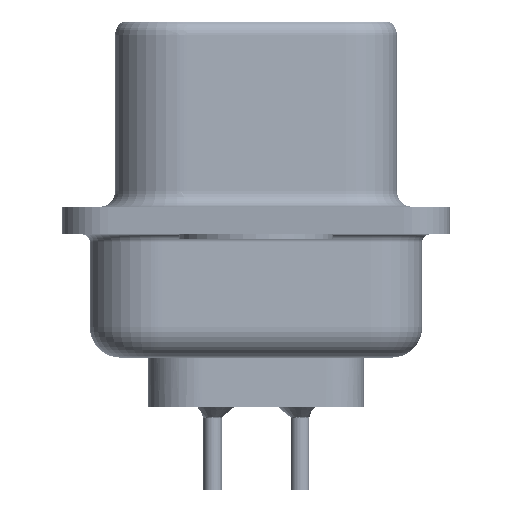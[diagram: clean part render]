
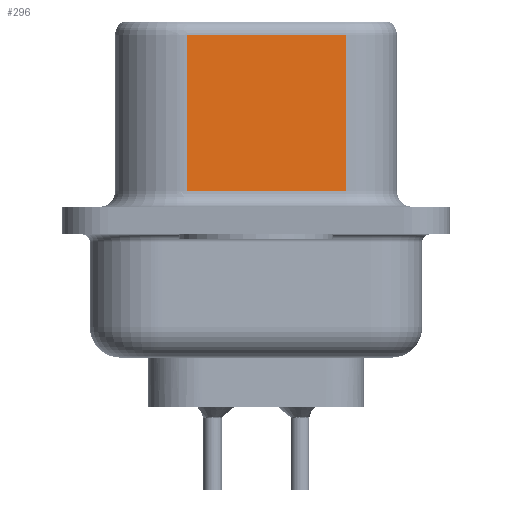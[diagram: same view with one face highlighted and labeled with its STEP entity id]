
A CAD part, left-side view. The second image highlights one B-rep face of the part: STEP entity #296.
In plain terms, the highlighted planar face has unit normal (-0.985, -0.174, 0).
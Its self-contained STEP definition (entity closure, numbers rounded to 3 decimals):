
#18 = EDGE_CURVE ( 'NONE', #11687, #7182, #13316, .T. ) ;
#296 = ADVANCED_FACE ( 'NONE', ( #2299 ), #26320, .F. ) ;
#1894 = CARTESIAN_POINT ( 'NONE',  ( 4.58, -2.927, 0.95 ) ) ;
#2299 = FACE_OUTER_BOUND ( 'NONE', #3265, .T. ) ;
#3113 = DIRECTION ( 'NONE',  ( 0., 0., -1. ) ) ;
#3265 = EDGE_LOOP ( 'NONE', ( #18052, #6284, #12231, #6590 ) ) ;
#4286 = CARTESIAN_POINT ( 'NONE',  ( 3.67, 2.233, 0.95 ) ) ;
#6068 = DIRECTION ( 'NONE',  ( 0.174, -0.985, 0. ) ) ;
#6284 = ORIENTED_EDGE ( 'NONE', *, *, #18, .T. ) ;
#6505 = LINE ( 'NONE', #22562, #27041 ) ;
#6590 = ORIENTED_EDGE ( 'NONE', *, *, #26422, .T. ) ;
#7182 = VERTEX_POINT ( 'NONE', #14924 ) ;
#7761 = VECTOR ( 'NONE', #12858, 1000. ) ;
#9754 = VERTEX_POINT ( 'NONE', #1894 ) ;
#10803 = AXIS2_PLACEMENT_3D ( 'NONE', #24267, #11584, #26406 ) ;
#11584 = DIRECTION ( 'NONE',  ( 0.985, 0.174, 0. ) ) ;
#11687 = VERTEX_POINT ( 'NONE', #21742 ) ;
#11847 = LINE ( 'NONE', #13691, #22468 ) ;
#12231 = ORIENTED_EDGE ( 'NONE', *, *, #18137, .T. ) ;
#12858 = DIRECTION ( 'NONE',  ( -0.174, 0.985, 0. ) ) ;
#13316 = LINE ( 'NONE', #16980, #7761 ) ;
#13575 = VECTOR ( 'NONE', #6068, 1000. ) ;
#13691 = CARTESIAN_POINT ( 'NONE',  ( 4.58, -2.927, 6.52 ) ) ;
#14443 = CARTESIAN_POINT ( 'NONE',  ( 4.58, -2.927, 0.95 ) ) ;
#14924 = CARTESIAN_POINT ( 'NONE',  ( 3.67, 2.233, 6.02 ) ) ;
#16980 = CARTESIAN_POINT ( 'NONE',  ( 4.58, -2.927, 6.02 ) ) ;
#18052 = ORIENTED_EDGE ( 'NONE', *, *, #21977, .F. ) ;
#18137 = EDGE_CURVE ( 'NONE', #7182, #27157, #6505, .T. ) ;
#19262 = LINE ( 'NONE', #14443, #13575 ) ;
#21742 = CARTESIAN_POINT ( 'NONE',  ( 4.58, -2.927, 6.02 ) ) ;
#21977 = EDGE_CURVE ( 'NONE', #11687, #9754, #11847, .T. ) ;
#22468 = VECTOR ( 'NONE', #3113, 1000. ) ;
#22562 = CARTESIAN_POINT ( 'NONE',  ( 3.67, 2.233, 6.52 ) ) ;
#24267 = CARTESIAN_POINT ( 'NONE',  ( 4.58, -2.927, 6.52 ) ) ;
#24668 = DIRECTION ( 'NONE',  ( 0., 0., -1. ) ) ;
#26320 = PLANE ( 'NONE',  #10803 ) ;
#26406 = DIRECTION ( 'NONE',  ( -0.174, 0.985, 0. ) ) ;
#26422 = EDGE_CURVE ( 'NONE', #27157, #9754, #19262, .T. ) ;
#27041 = VECTOR ( 'NONE', #24668, 1000. ) ;
#27157 = VERTEX_POINT ( 'NONE', #4286 ) ;
